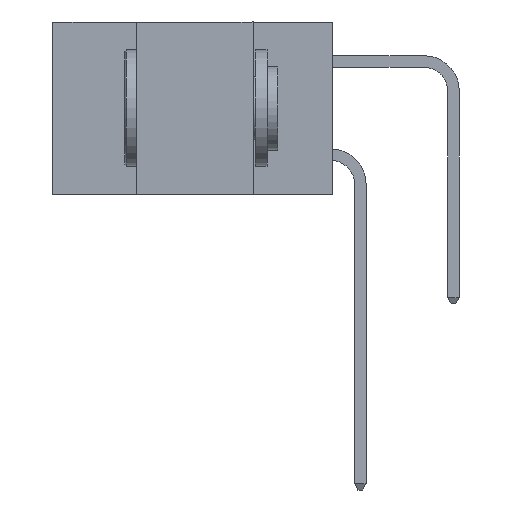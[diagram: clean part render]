
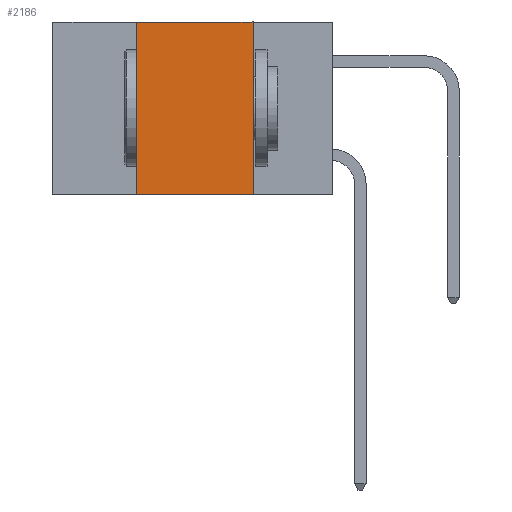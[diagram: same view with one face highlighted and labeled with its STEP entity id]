
A CAD part, left-side view. The second image highlights one B-rep face of the part: STEP entity #2186.
In plain terms, the highlighted planar face has unit normal (-1, 0, 0).
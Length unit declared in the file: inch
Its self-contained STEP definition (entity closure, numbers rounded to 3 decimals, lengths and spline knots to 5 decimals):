
#30 = AXIS2_PLACEMENT_3D ( 'NONE', #12803, #12627, #11214 ) ;
#873 = VECTOR ( 'NONE', #14839, 39.37008 ) ;
#1360 = CARTESIAN_POINT ( 'NONE',  ( 0., 0.17, -0.37 ) ) ;
#2186 = ADVANCED_FACE ( 'NONE', ( #5859 ), #9497, .F. ) ;
#3106 = VERTEX_POINT ( 'NONE', #12772 ) ;
#4080 = CARTESIAN_POINT ( 'NONE',  ( 0., 0.42, -0.37 ) ) ;
#4117 = DIRECTION ( 'NONE',  ( 0., 0., 1. ) ) ;
#4567 = LINE ( 'NONE', #4080, #7396 ) ;
#4718 = ORIENTED_EDGE ( 'NONE', *, *, #14980, .T. ) ;
#5140 = VECTOR ( 'NONE', #10470, 39.37008 ) ;
#5310 = VERTEX_POINT ( 'NONE', #1360 ) ;
#5515 = ORIENTED_EDGE ( 'NONE', *, *, #6772, .F. ) ;
#5736 = ORIENTED_EDGE ( 'NONE', *, *, #6221, .F. ) ;
#5859 = FACE_OUTER_BOUND ( 'NONE', #7733, .T. ) ;
#6221 = EDGE_CURVE ( 'NONE', #13708, #3106, #14809, .T. ) ;
#6581 = ORIENTED_EDGE ( 'NONE', *, *, #11726, .F. ) ;
#6772 = EDGE_CURVE ( 'NONE', #8407, #13708, #4567, .T. ) ;
#6937 = CARTESIAN_POINT ( 'NONE',  ( 0., 0.17, -0.37 ) ) ;
#7396 = VECTOR ( 'NONE', #4117, 39.37008 ) ;
#7733 = EDGE_LOOP ( 'NONE', ( #6581, #5736, #5515, #4718 ) ) ;
#8407 = VERTEX_POINT ( 'NONE', #14664 ) ;
#8853 = CARTESIAN_POINT ( 'NONE',  ( 0., 0.42, 0. ) ) ;
#9322 = CARTESIAN_POINT ( 'NONE',  ( 0., 0.6, -0.37 ) ) ;
#9497 = PLANE ( 'NONE',  #30 ) ;
#9937 = DIRECTION ( 'NONE',  ( 0., -1., 0. ) ) ;
#9970 = CARTESIAN_POINT ( 'NONE',  ( 0., 0.6, 0. ) ) ;
#10470 = DIRECTION ( 'NONE',  ( 0., -1., 0. ) ) ;
#11214 = DIRECTION ( 'NONE',  ( 0., 0., -1. ) ) ;
#11726 = EDGE_CURVE ( 'NONE', #3106, #5310, #13561, .T. ) ;
#12627 = DIRECTION ( 'NONE',  ( 1., 0., 0. ) ) ;
#12772 = CARTESIAN_POINT ( 'NONE',  ( 0., 0.17, 0. ) ) ;
#12803 = CARTESIAN_POINT ( 'NONE',  ( 0., 0.6, 0. ) ) ;
#13561 = LINE ( 'NONE', #6937, #873 ) ;
#13708 = VERTEX_POINT ( 'NONE', #8853 ) ;
#13962 = LINE ( 'NONE', #9322, #5140 ) ;
#14502 = VECTOR ( 'NONE', #9937, 39.37008 ) ;
#14664 = CARTESIAN_POINT ( 'NONE',  ( 0., 0.42, -0.37 ) ) ;
#14809 = LINE ( 'NONE', #9970, #14502 ) ;
#14839 = DIRECTION ( 'NONE',  ( 0., 0., -1. ) ) ;
#14980 = EDGE_CURVE ( 'NONE', #8407, #5310, #13962, .T. ) ;
